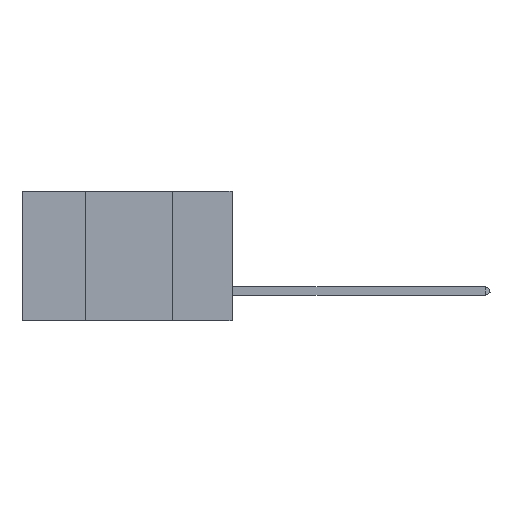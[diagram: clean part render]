
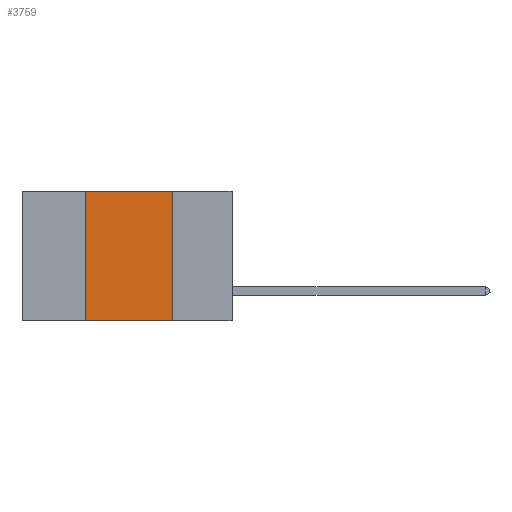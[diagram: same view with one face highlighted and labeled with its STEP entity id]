
A CAD part, left-side view. The second image highlights one B-rep face of the part: STEP entity #3759.
In plain terms, the highlighted planar face has unit normal (-1, 0, 0).
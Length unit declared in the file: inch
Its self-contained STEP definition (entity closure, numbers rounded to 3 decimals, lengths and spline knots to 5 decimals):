
#236 = VECTOR ( 'NONE', #2947, 39.37008 ) ;
#381 = DIRECTION ( 'NONE',  ( 0., 0., -1. ) ) ;
#403 = ORIENTED_EDGE ( 'NONE', *, *, #9462, .F. ) ;
#1216 = CARTESIAN_POINT ( 'NONE',  ( 0., 0.42, -0.37 ) ) ;
#2425 = DIRECTION ( 'NONE',  ( 1., 0., 0. ) ) ;
#2947 = DIRECTION ( 'NONE',  ( 0., -1., 0. ) ) ;
#3007 = LINE ( 'NONE', #6963, #10130 ) ;
#3218 = DIRECTION ( 'NONE',  ( 0., -1., 0. ) ) ;
#3234 = ORIENTED_EDGE ( 'NONE', *, *, #7593, .T. ) ;
#3672 = CARTESIAN_POINT ( 'NONE',  ( 0., 0.42, 0. ) ) ;
#3737 = VERTEX_POINT ( 'NONE', #3672 ) ;
#3759 = ADVANCED_FACE ( 'NONE', ( #8335 ), #4637, .F. ) ;
#3769 = EDGE_CURVE ( 'NONE', #3737, #5095, #4489, .T. ) ;
#3829 = LINE ( 'NONE', #8396, #11300 ) ;
#4159 = EDGE_CURVE ( 'NONE', #5095, #8631, #3007, .T. ) ;
#4489 = LINE ( 'NONE', #9613, #12679 ) ;
#4637 = PLANE ( 'NONE',  #5513 ) ;
#5095 = VERTEX_POINT ( 'NONE', #12020 ) ;
#5513 = AXIS2_PLACEMENT_3D ( 'NONE', #11973, #2425, #381 ) ;
#6541 = EDGE_LOOP ( 'NONE', ( #12288, #11279, #403, #3234 ) ) ;
#6963 = CARTESIAN_POINT ( 'NONE',  ( 0., 0.17, 0. ) ) ;
#7018 = CARTESIAN_POINT ( 'NONE',  ( 0., 0.6, -0.37 ) ) ;
#7593 = EDGE_CURVE ( 'NONE', #10290, #8631, #10864, .T. ) ;
#8023 = DIRECTION ( 'NONE',  ( 0., 0., -1. ) ) ;
#8335 = FACE_OUTER_BOUND ( 'NONE', #6541, .T. ) ;
#8396 = CARTESIAN_POINT ( 'NONE',  ( 0., 0.42, 0. ) ) ;
#8631 = VERTEX_POINT ( 'NONE', #11753 ) ;
#9462 = EDGE_CURVE ( 'NONE', #10290, #3737, #3829, .T. ) ;
#9613 = CARTESIAN_POINT ( 'NONE',  ( 0., 0.6, 0. ) ) ;
#10130 = VECTOR ( 'NONE', #8023, 39.37008 ) ;
#10290 = VERTEX_POINT ( 'NONE', #1216 ) ;
#10864 = LINE ( 'NONE', #7018, #236 ) ;
#11279 = ORIENTED_EDGE ( 'NONE', *, *, #3769, .F. ) ;
#11300 = VECTOR ( 'NONE', #12748, 39.37008 ) ;
#11753 = CARTESIAN_POINT ( 'NONE',  ( 0., 0.17, -0.37 ) ) ;
#11973 = CARTESIAN_POINT ( 'NONE',  ( 0., 0.6, 0. ) ) ;
#12020 = CARTESIAN_POINT ( 'NONE',  ( 0., 0.17, 0. ) ) ;
#12288 = ORIENTED_EDGE ( 'NONE', *, *, #4159, .F. ) ;
#12679 = VECTOR ( 'NONE', #3218, 39.37008 ) ;
#12748 = DIRECTION ( 'NONE',  ( 0., 0., 1. ) ) ;
